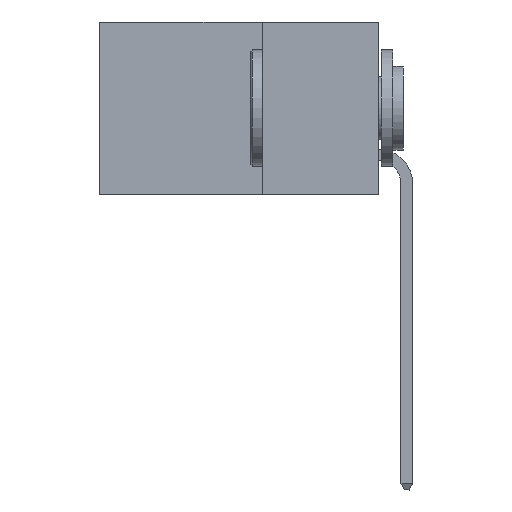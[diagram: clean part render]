
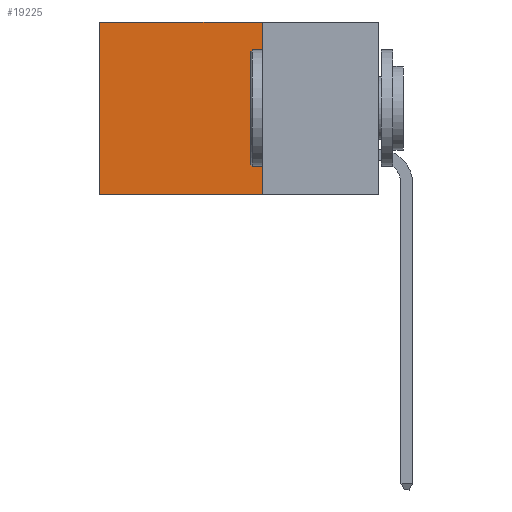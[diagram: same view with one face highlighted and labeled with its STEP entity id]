
A CAD part, left-side view. The second image highlights one B-rep face of the part: STEP entity #19225.
In plain terms, the highlighted planar face has unit normal (-1, 0, 0).
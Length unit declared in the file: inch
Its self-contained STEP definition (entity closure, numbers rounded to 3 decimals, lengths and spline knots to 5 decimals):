
#1493 = DIRECTION ( 'NONE',  ( 0., 0., -1. ) ) ;
#1755 = EDGE_LOOP ( 'NONE', ( #5022, #15740, #18851, #12557 ) ) ;
#2363 = CARTESIAN_POINT ( 'NONE',  ( 0.298, 0.6, -0.37 ) ) ;
#2662 = VERTEX_POINT ( 'NONE', #2363 ) ;
#4293 = AXIS2_PLACEMENT_3D ( 'NONE', #16704, #4685, #15313 ) ;
#4685 = DIRECTION ( 'NONE',  ( 1., 0., 0. ) ) ;
#5022 = ORIENTED_EDGE ( 'NONE', *, *, #7167, .T. ) ;
#5409 = LINE ( 'NONE', #10637, #17400 ) ;
#5679 = CARTESIAN_POINT ( 'NONE',  ( 0.298, 0.25, -0.37 ) ) ;
#6095 = EDGE_CURVE ( 'NONE', #8939, #8362, #5409, .T. ) ;
#6800 = EDGE_CURVE ( 'NONE', #6990, #2662, #13401, .T. ) ;
#6990 = VERTEX_POINT ( 'NONE', #5679 ) ;
#7167 = EDGE_CURVE ( 'NONE', #8362, #2662, #13850, .T. ) ;
#7628 = CARTESIAN_POINT ( 'NONE',  ( 0.298, 0.6, 0. ) ) ;
#8362 = VERTEX_POINT ( 'NONE', #7628 ) ;
#8939 = VERTEX_POINT ( 'NONE', #13456 ) ;
#9309 = CARTESIAN_POINT ( 'NONE',  ( 0.298, 0.6, 0. ) ) ;
#9928 = VECTOR ( 'NONE', #12311, 39.37008 ) ;
#10637 = CARTESIAN_POINT ( 'NONE',  ( 0.298, 0.25, 0. ) ) ;
#10770 = CARTESIAN_POINT ( 'NONE',  ( 0.298, 0.25, 0. ) ) ;
#12311 = DIRECTION ( 'NONE',  ( 0., 0., -1. ) ) ;
#12360 = PLANE ( 'NONE',  #4293 ) ;
#12557 = ORIENTED_EDGE ( 'NONE', *, *, #6095, .T. ) ;
#12760 = DIRECTION ( 'NONE',  ( 0., 1., 0. ) ) ;
#13401 = LINE ( 'NONE', #18877, #16838 ) ;
#13456 = CARTESIAN_POINT ( 'NONE',  ( 0.298, 0.25, 0. ) ) ;
#13622 = EDGE_CURVE ( 'NONE', #8939, #6990, #18198, .T. ) ;
#13822 = VECTOR ( 'NONE', #1493, 39.37008 ) ;
#13850 = LINE ( 'NONE', #9309, #9928 ) ;
#14791 = DIRECTION ( 'NONE',  ( 0., 1., 0. ) ) ;
#15178 = FACE_OUTER_BOUND ( 'NONE', #1755, .T. ) ;
#15313 = DIRECTION ( 'NONE',  ( 0., 0., -1. ) ) ;
#15740 = ORIENTED_EDGE ( 'NONE', *, *, #6800, .F. ) ;
#16704 = CARTESIAN_POINT ( 'NONE',  ( 0.298, 0.25, 0. ) ) ;
#16838 = VECTOR ( 'NONE', #14791, 39.37008 ) ;
#17400 = VECTOR ( 'NONE', #12760, 39.37008 ) ;
#18198 = LINE ( 'NONE', #10770, #13822 ) ;
#18851 = ORIENTED_EDGE ( 'NONE', *, *, #13622, .F. ) ;
#18877 = CARTESIAN_POINT ( 'NONE',  ( 0.298, 0.25, -0.37 ) ) ;
#19225 = ADVANCED_FACE ( 'NONE', ( #15178 ), #12360, .F. ) ;
